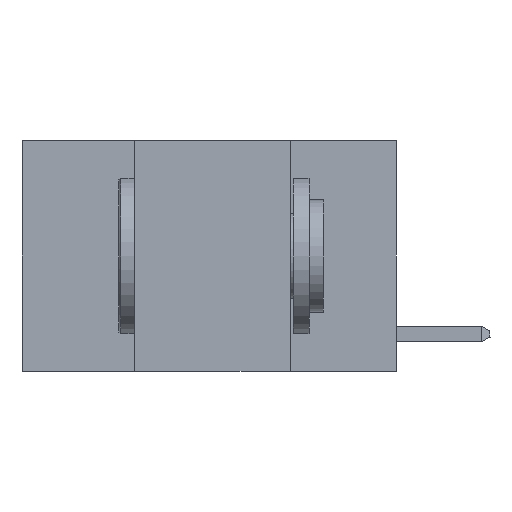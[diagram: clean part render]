
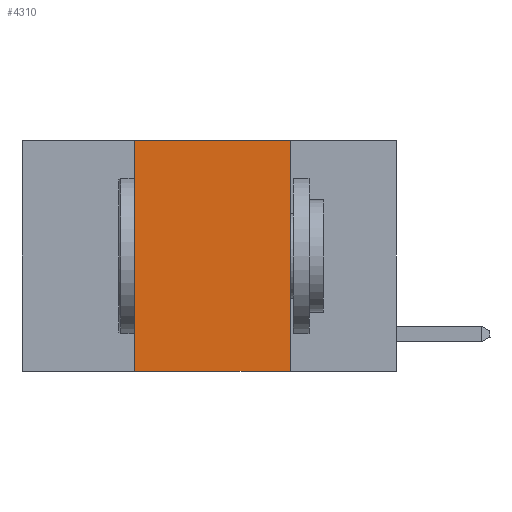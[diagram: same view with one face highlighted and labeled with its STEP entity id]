
A CAD part, left-side view. The second image highlights one B-rep face of the part: STEP entity #4310.
In plain terms, the highlighted planar face has unit normal (-1, 0, 0).
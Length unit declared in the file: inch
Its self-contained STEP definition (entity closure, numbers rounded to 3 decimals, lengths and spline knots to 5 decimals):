
#708 = CARTESIAN_POINT ( 'NONE',  ( 0., 0.17, -0.37 ) ) ;
#1488 = CARTESIAN_POINT ( 'NONE',  ( 0., 0.6, -0.37 ) ) ;
#4246 = FACE_OUTER_BOUND ( 'NONE', #22688, .T. ) ;
#4310 = ADVANCED_FACE ( 'NONE', ( #4246 ), #6585, .F. ) ;
#4484 = LINE ( 'NONE', #19037, #8376 ) ;
#5403 = EDGE_CURVE ( 'NONE', #6980, #22693, #21810, .T. ) ;
#5593 = CARTESIAN_POINT ( 'NONE',  ( 0., 0.6, 0. ) ) ;
#5778 = DIRECTION ( 'NONE',  ( 0., 0., 1. ) ) ;
#6545 = CARTESIAN_POINT ( 'NONE',  ( 0., 0.17, 0. ) ) ;
#6585 = PLANE ( 'NONE',  #21726 ) ;
#6980 = VERTEX_POINT ( 'NONE', #7861 ) ;
#7861 = CARTESIAN_POINT ( 'NONE',  ( 0., 0.42, 0. ) ) ;
#7983 = VERTEX_POINT ( 'NONE', #708 ) ;
#8376 = VECTOR ( 'NONE', #10003, 39.37008 ) ;
#8610 = ORIENTED_EDGE ( 'NONE', *, *, #5403, .F. ) ;
#8698 = DIRECTION ( 'NONE',  ( 0., -1., 0. ) ) ;
#8994 = VERTEX_POINT ( 'NONE', #19682 ) ;
#9887 = DIRECTION ( 'NONE',  ( 1., 0., 0. ) ) ;
#10003 = DIRECTION ( 'NONE',  ( 0., 0., -1. ) ) ;
#10804 = EDGE_CURVE ( 'NONE', #8994, #6980, #14755, .T. ) ;
#10944 = ORIENTED_EDGE ( 'NONE', *, *, #22250, .T. ) ;
#11876 = VECTOR ( 'NONE', #14797, 39.37008 ) ;
#12609 = CARTESIAN_POINT ( 'NONE',  ( 0., 0.42, 0. ) ) ;
#13879 = LINE ( 'NONE', #1488, #18944 ) ;
#14755 = LINE ( 'NONE', #12609, #22071 ) ;
#14797 = DIRECTION ( 'NONE',  ( 0., -1., 0. ) ) ;
#15508 = EDGE_CURVE ( 'NONE', #22693, #7983, #4484, .T. ) ;
#17009 = DIRECTION ( 'NONE',  ( 0., 0., -1. ) ) ;
#17142 = ORIENTED_EDGE ( 'NONE', *, *, #10804, .F. ) ;
#18944 = VECTOR ( 'NONE', #8698, 39.37008 ) ;
#19037 = CARTESIAN_POINT ( 'NONE',  ( 0., 0.17, 0. ) ) ;
#19682 = CARTESIAN_POINT ( 'NONE',  ( 0., 0.42, -0.37 ) ) ;
#21726 = AXIS2_PLACEMENT_3D ( 'NONE', #22590, #9887, #17009 ) ;
#21810 = LINE ( 'NONE', #5593, #11876 ) ;
#22071 = VECTOR ( 'NONE', #5778, 39.37008 ) ;
#22250 = EDGE_CURVE ( 'NONE', #8994, #7983, #13879, .T. ) ;
#22590 = CARTESIAN_POINT ( 'NONE',  ( 0., 0.6, 0. ) ) ;
#22688 = EDGE_LOOP ( 'NONE', ( #22839, #8610, #17142, #10944 ) ) ;
#22693 = VERTEX_POINT ( 'NONE', #6545 ) ;
#22839 = ORIENTED_EDGE ( 'NONE', *, *, #15508, .F. ) ;
